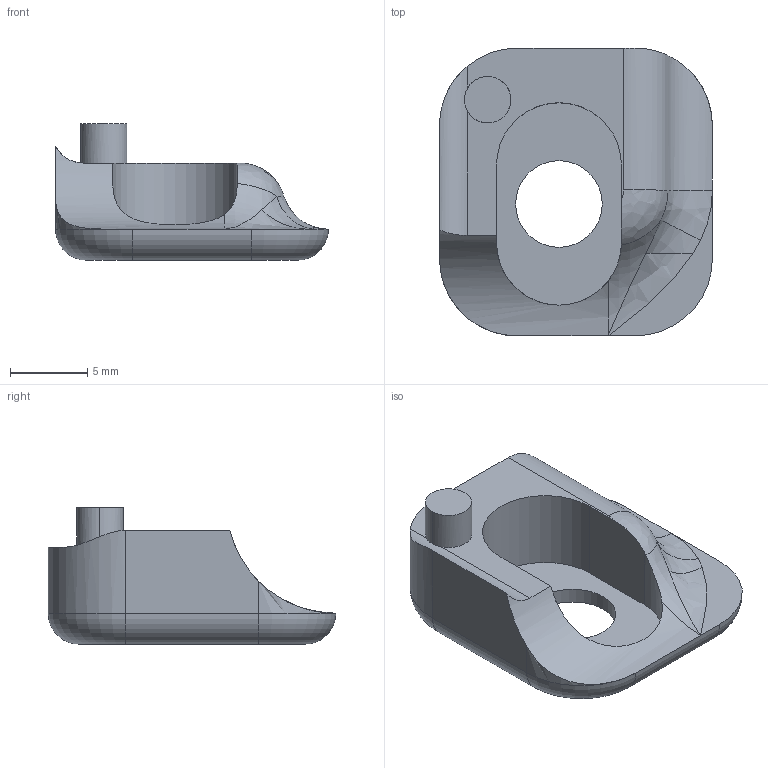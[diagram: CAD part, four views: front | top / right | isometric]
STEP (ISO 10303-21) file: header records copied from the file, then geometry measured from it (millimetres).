
FILE_DESCRIPTION (( 'STEP AP214' ), '1' );
FILE_NAME ('CharonFCG_Release_Cover.STEP', '2013-12-17T06:09:33', ( 'elpi' ), ( '' ), 'SwSTEP 2.0', 'SolidWorks 2013', '' );
FILE_SCHEMA (( 'AUTOMOTIVE_DESIGN' ));
Length unit declared in the file: inch
Products named in the file (1): CharonFCG_Release_Cover
Bounding box: 17.64 x 18.6 x 8.82 mm (x, y, z)
Volume: 981.4 mm3; surface area: 984.3 mm2
Topology: 1 solids, 1 shells, 36 faces, 92 edges, 57 vertices
Faces by surface type: cylinder 18, plane 9, torus 5, bspline 4
Entity records: 1403 total; most frequent: CARTESIAN_POINT 521, ORIENTED_EDGE 182, DIRECTION 172, EDGE_CURVE 91, AXIS2_PLACEMENT_3D 69, VERTEX_POINT 57, EDGE_LOOP 38, FACE_OUTER_BOUND 36
